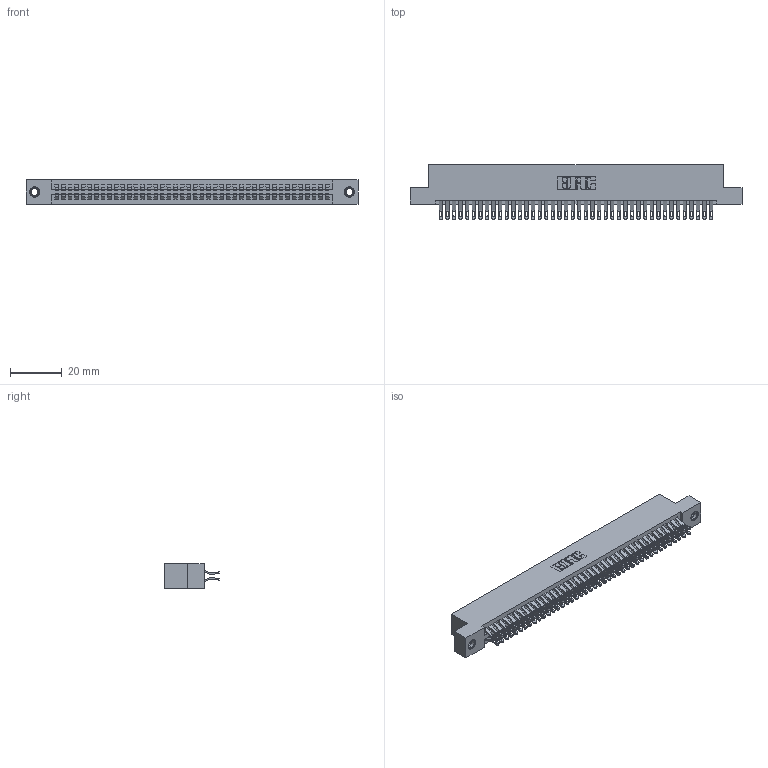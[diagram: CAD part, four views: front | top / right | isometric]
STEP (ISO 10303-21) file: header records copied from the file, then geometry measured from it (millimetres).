
FILE_DESCRIPTION (( 'STEP AP203' ), '1' );
FILE_NAME ('395-084-555-207.STEP', '2018-11-28T15:45:34', ( '' ), ( '' ), 'SwSTEP 2.0', 'SolidWorks 2016', '' );
FILE_SCHEMA (( 'CONFIG_CONTROL_DESIGN' ));
Length unit declared in the file: inch
Products named in the file (4): 345-250-001_345-250-005-103; 395-084-555-207; 345-292-001_555 Tail; 345 Part_Flush Mounting Lugs - 0.156 Dia-TI
Assembly tree (87 placements, depth 2):
  395-084-555-207
    345 Part_Flush Mounting Lugs - 0.156 Dia-TI
    345-292-001_555 Tail  x84
    345-250-001_345-250-005-103  x2
Bounding box: 127.89 x 21.13 x 9.4 mm (x, y, z)
Volume: 12653.4 mm3; surface area: 19579.2 mm2
Topology: 87 solids, 87 shells, 4890 faces, 15345 edges, 10222 vertices
Faces by surface type: plane 2716, cylinder 2158, cone 12, torus 4
Entity records: 34466 total; most frequent: CARTESIAN_POINT 5793, ORIENTED_EDGE 5690, DIRECTION 5103, EDGE_CURVE 2845, LINE 2505, VECTOR 2505, VERTEX_POINT 1892, AXIS2_PLACEMENT_3D 1299
